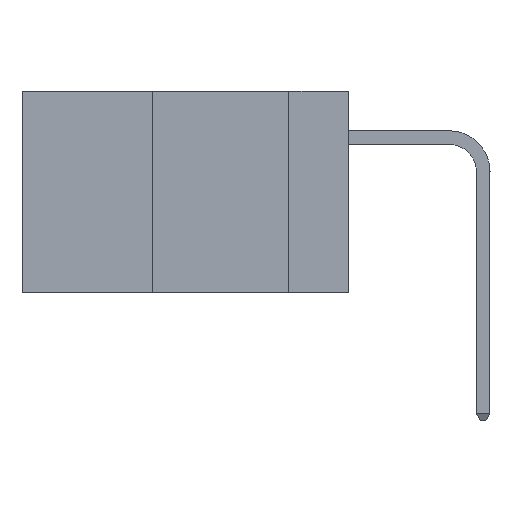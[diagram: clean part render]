
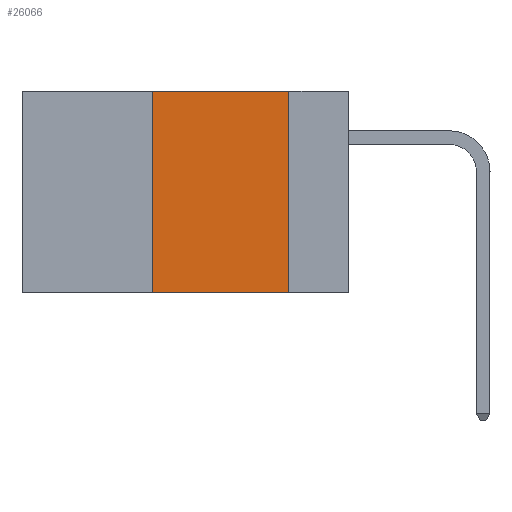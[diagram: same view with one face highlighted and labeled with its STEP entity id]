
A CAD part, left-side view. The second image highlights one B-rep face of the part: STEP entity #26066.
In plain terms, the highlighted planar face has unit normal (-1, 0, 0).
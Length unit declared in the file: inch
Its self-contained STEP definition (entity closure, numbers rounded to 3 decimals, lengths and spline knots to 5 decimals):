
#45 = VERTEX_POINT ( 'NONE', #25064 ) ;
#1477 = VERTEX_POINT ( 'NONE', #32941 ) ;
#1564 = AXIS2_PLACEMENT_3D ( 'NONE', #14215, #34739, #11282 ) ;
#1628 = DIRECTION ( 'NONE',  ( 0., 0., 1. ) ) ;
#2198 = CARTESIAN_POINT ( 'NONE',  ( 0., 0.36, 0. ) ) ;
#3031 = ORIENTED_EDGE ( 'NONE', *, *, #9010, .T. ) ;
#4154 = LINE ( 'NONE', #17584, #42491 ) ;
#6699 = DIRECTION ( 'NONE',  ( 0., -1., 0. ) ) ;
#9010 = EDGE_CURVE ( 'NONE', #11696, #13072, #4154, .T. ) ;
#9137 = CARTESIAN_POINT ( 'NONE',  ( 0., 0.11, -0.37 ) ) ;
#11282 = DIRECTION ( 'NONE',  ( 0., 0., -1. ) ) ;
#11696 = VERTEX_POINT ( 'NONE', #17719 ) ;
#12238 = CARTESIAN_POINT ( 'NONE',  ( 0., 0.11, 0. ) ) ;
#12939 = VECTOR ( 'NONE', #1628, 39.37008 ) ;
#13072 = VERTEX_POINT ( 'NONE', #9137 ) ;
#14081 = ORIENTED_EDGE ( 'NONE', *, *, #38223, .F. ) ;
#14215 = CARTESIAN_POINT ( 'NONE',  ( 0., 0.6, 0. ) ) ;
#14358 = VECTOR ( 'NONE', #14709, 39.37008 ) ;
#14709 = DIRECTION ( 'NONE',  ( 0., -1., 0. ) ) ;
#17058 = ORIENTED_EDGE ( 'NONE', *, *, #34600, .F. ) ;
#17584 = CARTESIAN_POINT ( 'NONE',  ( 0., 0.6, -0.37 ) ) ;
#17719 = CARTESIAN_POINT ( 'NONE',  ( 0., 0.36, -0.37 ) ) ;
#20244 = LINE ( 'NONE', #2198, #12939 ) ;
#25049 = EDGE_LOOP ( 'NONE', ( #17058, #29951, #14081, #3031 ) ) ;
#25064 = CARTESIAN_POINT ( 'NONE',  ( 0., 0.36, 0. ) ) ;
#25693 = LINE ( 'NONE', #12238, #31997 ) ;
#26066 = ADVANCED_FACE ( 'NONE', ( #42362 ), #40936, .F. ) ;
#28522 = EDGE_CURVE ( 'NONE', #45, #1477, #32719, .T. ) ;
#29951 = ORIENTED_EDGE ( 'NONE', *, *, #28522, .F. ) ;
#31997 = VECTOR ( 'NONE', #35707, 39.37008 ) ;
#32719 = LINE ( 'NONE', #38057, #14358 ) ;
#32941 = CARTESIAN_POINT ( 'NONE',  ( 0., 0.11, 0. ) ) ;
#34600 = EDGE_CURVE ( 'NONE', #1477, #13072, #25693, .T. ) ;
#34739 = DIRECTION ( 'NONE',  ( 1., 0., 0. ) ) ;
#35707 = DIRECTION ( 'NONE',  ( 0., 0., -1. ) ) ;
#38057 = CARTESIAN_POINT ( 'NONE',  ( 0., 0.6, 0. ) ) ;
#38223 = EDGE_CURVE ( 'NONE', #11696, #45, #20244, .T. ) ;
#40936 = PLANE ( 'NONE',  #1564 ) ;
#42362 = FACE_OUTER_BOUND ( 'NONE', #25049, .T. ) ;
#42491 = VECTOR ( 'NONE', #6699, 39.37008 ) ;
